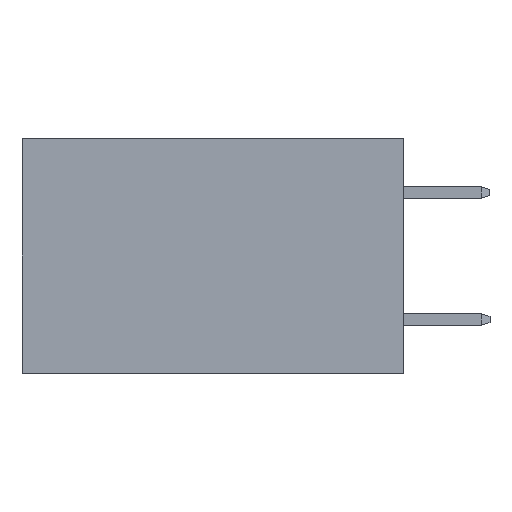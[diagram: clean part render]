
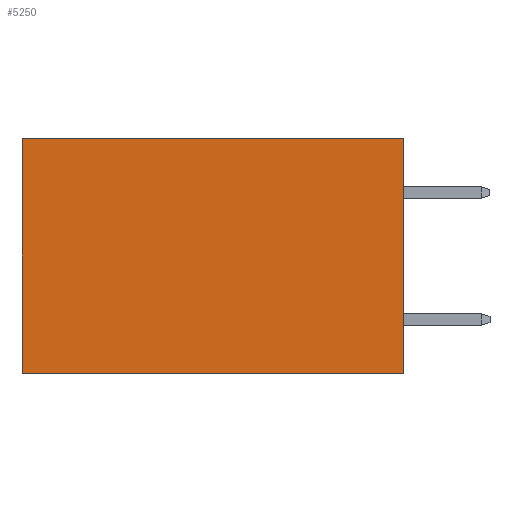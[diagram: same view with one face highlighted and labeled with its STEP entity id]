
A CAD part, left-side view. The second image highlights one B-rep face of the part: STEP entity #5250.
In plain terms, the highlighted planar face has unit normal (-1, 0, 0).
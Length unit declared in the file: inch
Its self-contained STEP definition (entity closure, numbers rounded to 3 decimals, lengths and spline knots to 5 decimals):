
#87 = DIRECTION ( 'NONE',  ( 0., 1., 0. ) ) ;
#163 = DIRECTION ( 'NONE',  ( 1., 0., 0. ) ) ;
#209 = CARTESIAN_POINT ( 'NONE',  ( 0.2875, 0., 0. ) ) ;
#485 = VECTOR ( 'NONE', #2756, 39.37008 ) ;
#686 = VECTOR ( 'NONE', #3604, 39.37008 ) ;
#796 = EDGE_LOOP ( 'NONE', ( #4277, #3573, #2954, #7734 ) ) ;
#1431 = CARTESIAN_POINT ( 'NONE',  ( 0.2875, 0.6, -0.37 ) ) ;
#1540 = FACE_OUTER_BOUND ( 'NONE', #796, .T. ) ;
#1566 = EDGE_CURVE ( 'NONE', #6002, #3894, #4971, .T. ) ;
#2027 = VECTOR ( 'NONE', #4195, 39.37008 ) ;
#2167 = LINE ( 'NONE', #2693, #2537 ) ;
#2226 = CARTESIAN_POINT ( 'NONE',  ( 0.2875, 0.6, 0. ) ) ;
#2522 = AXIS2_PLACEMENT_3D ( 'NONE', #209, #163, #7596 ) ;
#2537 = VECTOR ( 'NONE', #87, 39.37008 ) ;
#2693 = CARTESIAN_POINT ( 'NONE',  ( 0.2875, 0., 0. ) ) ;
#2746 = CARTESIAN_POINT ( 'NONE',  ( 0.2875, 0., -0.37 ) ) ;
#2756 = DIRECTION ( 'NONE',  ( 0., 0., -1. ) ) ;
#2803 = CARTESIAN_POINT ( 'NONE',  ( 0.2875, 0., 0. ) ) ;
#2954 = ORIENTED_EDGE ( 'NONE', *, *, #1566, .F. ) ;
#3254 = EDGE_CURVE ( 'NONE', #7078, #8146, #5950, .T. ) ;
#3573 = ORIENTED_EDGE ( 'NONE', *, *, #3715, .F. ) ;
#3604 = DIRECTION ( 'NONE',  ( 0., 0., -1. ) ) ;
#3715 = EDGE_CURVE ( 'NONE', #3894, #8146, #7530, .T. ) ;
#3894 = VERTEX_POINT ( 'NONE', #7164 ) ;
#4195 = DIRECTION ( 'NONE',  ( 0., 1., 0. ) ) ;
#4277 = ORIENTED_EDGE ( 'NONE', *, *, #3254, .T. ) ;
#4971 = LINE ( 'NONE', #8292, #686 ) ;
#5250 = ADVANCED_FACE ( 'NONE', ( #1540 ), #5559, .F. ) ;
#5559 = PLANE ( 'NONE',  #2522 ) ;
#5950 = LINE ( 'NONE', #2226, #485 ) ;
#6002 = VERTEX_POINT ( 'NONE', #2803 ) ;
#7078 = VERTEX_POINT ( 'NONE', #8084 ) ;
#7164 = CARTESIAN_POINT ( 'NONE',  ( 0.2875, 0., -0.37 ) ) ;
#7530 = LINE ( 'NONE', #2746, #2027 ) ;
#7596 = DIRECTION ( 'NONE',  ( 0., 0., -1. ) ) ;
#7734 = ORIENTED_EDGE ( 'NONE', *, *, #8601, .T. ) ;
#8084 = CARTESIAN_POINT ( 'NONE',  ( 0.2875, 0.6, 0. ) ) ;
#8146 = VERTEX_POINT ( 'NONE', #1431 ) ;
#8292 = CARTESIAN_POINT ( 'NONE',  ( 0.2875, 0., 0. ) ) ;
#8601 = EDGE_CURVE ( 'NONE', #6002, #7078, #2167, .T. ) ;
